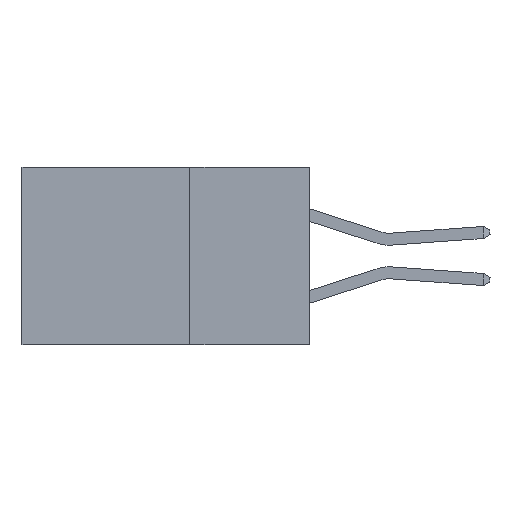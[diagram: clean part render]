
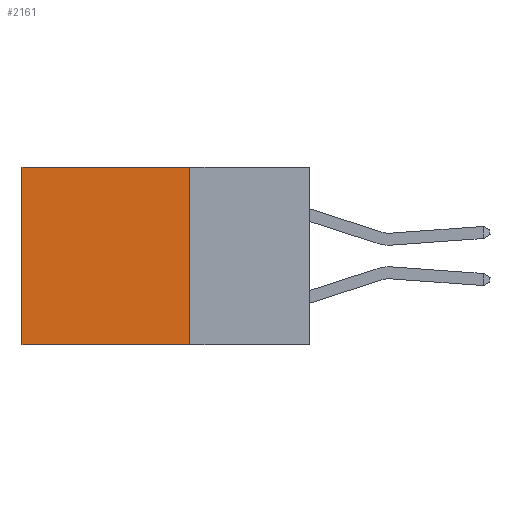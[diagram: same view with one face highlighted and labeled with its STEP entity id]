
A CAD part, left-side view. The second image highlights one B-rep face of the part: STEP entity #2161.
In plain terms, the highlighted planar face has unit normal (-1, 0, 0).
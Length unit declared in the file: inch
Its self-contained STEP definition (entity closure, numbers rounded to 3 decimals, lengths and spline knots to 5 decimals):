
#24 = DIRECTION ( 'NONE',  ( 1., 0., 0. ) ) ;
#26 = LINE ( 'NONE', #11300, #2886 ) ;
#699 = CARTESIAN_POINT ( 'NONE',  ( 0.298, 0.6, -0.37 ) ) ;
#1019 = ORIENTED_EDGE ( 'NONE', *, *, #8198, .F. ) ;
#1770 = DIRECTION ( 'NONE',  ( 0., 1., 0. ) ) ;
#2161 = ADVANCED_FACE ( 'NONE', ( #5156 ), #3190, .F. ) ;
#2193 = ORIENTED_EDGE ( 'NONE', *, *, #9436, .T. ) ;
#2530 = VECTOR ( 'NONE', #1770, 39.37008 ) ;
#2555 = AXIS2_PLACEMENT_3D ( 'NONE', #9167, #24, #3148 ) ;
#2689 = LINE ( 'NONE', #5821, #2530 ) ;
#2886 = VECTOR ( 'NONE', #5549, 39.37008 ) ;
#3148 = DIRECTION ( 'NONE',  ( 0., 0., -1. ) ) ;
#3190 = PLANE ( 'NONE',  #2555 ) ;
#3343 = EDGE_CURVE ( 'NONE', #7002, #9545, #12672, .T. ) ;
#3353 = ORIENTED_EDGE ( 'NONE', *, *, #3343, .F. ) ;
#3483 = VECTOR ( 'NONE', #10375, 39.37008 ) ;
#3973 = EDGE_CURVE ( 'NONE', #12626, #11449, #2689, .T. ) ;
#5156 = FACE_OUTER_BOUND ( 'NONE', #7511, .T. ) ;
#5482 = CARTESIAN_POINT ( 'NONE',  ( 0.298, 0.6, 0. ) ) ;
#5549 = DIRECTION ( 'NONE',  ( 0., 0., -1. ) ) ;
#5821 = CARTESIAN_POINT ( 'NONE',  ( 0.298, 0.25, 0. ) ) ;
#5907 = VECTOR ( 'NONE', #6800, 39.37008 ) ;
#6056 = CARTESIAN_POINT ( 'NONE',  ( 0.298, 0.25, 0. ) ) ;
#6800 = DIRECTION ( 'NONE',  ( 0., 1., 0. ) ) ;
#7002 = VERTEX_POINT ( 'NONE', #10030 ) ;
#7511 = EDGE_LOOP ( 'NONE', ( #2193, #3353, #1019, #12674 ) ) ;
#8198 = EDGE_CURVE ( 'NONE', #12626, #7002, #26, .T. ) ;
#9167 = CARTESIAN_POINT ( 'NONE',  ( 0.298, 0.25, 0. ) ) ;
#9436 = EDGE_CURVE ( 'NONE', #11449, #9545, #11835, .T. ) ;
#9545 = VERTEX_POINT ( 'NONE', #699 ) ;
#10030 = CARTESIAN_POINT ( 'NONE',  ( 0.298, 0.25, -0.37 ) ) ;
#10375 = DIRECTION ( 'NONE',  ( 0., 0., -1. ) ) ;
#11034 = CARTESIAN_POINT ( 'NONE',  ( 0.298, 0.25, -0.37 ) ) ;
#11300 = CARTESIAN_POINT ( 'NONE',  ( 0.298, 0.25, 0. ) ) ;
#11449 = VERTEX_POINT ( 'NONE', #5482 ) ;
#11835 = LINE ( 'NONE', #12627, #3483 ) ;
#12626 = VERTEX_POINT ( 'NONE', #6056 ) ;
#12627 = CARTESIAN_POINT ( 'NONE',  ( 0.298, 0.6, 0. ) ) ;
#12672 = LINE ( 'NONE', #11034, #5907 ) ;
#12674 = ORIENTED_EDGE ( 'NONE', *, *, #3973, .T. ) ;
